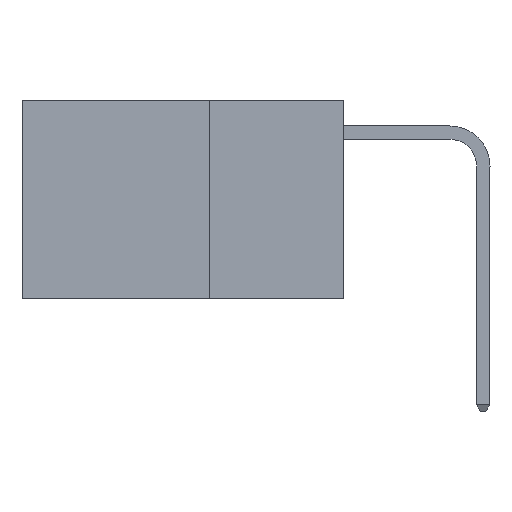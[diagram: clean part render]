
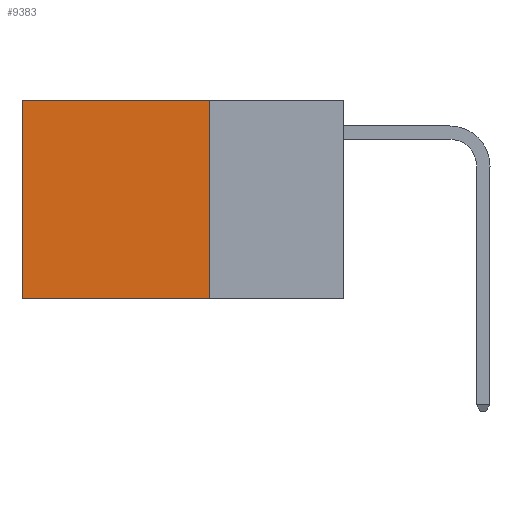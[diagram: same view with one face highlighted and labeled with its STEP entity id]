
A CAD part, left-side view. The second image highlights one B-rep face of the part: STEP entity #9383.
In plain terms, the highlighted planar face has unit normal (-1, 0, 0).
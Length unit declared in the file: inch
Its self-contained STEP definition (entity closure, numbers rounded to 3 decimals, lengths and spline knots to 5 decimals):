
#679 = CARTESIAN_POINT ( 'NONE',  ( 0.2625, 0.25, -0.37 ) ) ;
#1135 = VECTOR ( 'NONE', #7109, 39.37008 ) ;
#1164 = VERTEX_POINT ( 'NONE', #5361 ) ;
#1735 = DIRECTION ( 'NONE',  ( 0., 1., 0. ) ) ;
#1795 = CARTESIAN_POINT ( 'NONE',  ( 0.2625, 0.25, 0. ) ) ;
#3793 = ORIENTED_EDGE ( 'NONE', *, *, #11701, .F. ) ;
#4060 = VECTOR ( 'NONE', #1735, 39.37008 ) ;
#4200 = CARTESIAN_POINT ( 'NONE',  ( 0.2625, 0.25, -0.37 ) ) ;
#4463 = CARTESIAN_POINT ( 'NONE',  ( 0.2625, 0.25, 0. ) ) ;
#4546 = ORIENTED_EDGE ( 'NONE', *, *, #11304, .T. ) ;
#4791 = LINE ( 'NONE', #1795, #4060 ) ;
#5361 = CARTESIAN_POINT ( 'NONE',  ( 0.2625, 0.6, -0.37 ) ) ;
#5553 = CARTESIAN_POINT ( 'NONE',  ( 0.2625, 0.6, 0. ) ) ;
#5702 = FACE_OUTER_BOUND ( 'NONE', #10223, .T. ) ;
#5742 = PLANE ( 'NONE',  #12553 ) ;
#6445 = LINE ( 'NONE', #14404, #10274 ) ;
#7109 = DIRECTION ( 'NONE',  ( 0., 0., -1. ) ) ;
#7186 = CARTESIAN_POINT ( 'NONE',  ( 0.2625, 0.25, 0. ) ) ;
#7611 = VERTEX_POINT ( 'NONE', #5553 ) ;
#7677 = VECTOR ( 'NONE', #11231, 39.37008 ) ;
#7749 = LINE ( 'NONE', #4200, #7677 ) ;
#8507 = DIRECTION ( 'NONE',  ( 1., 0., 0. ) ) ;
#8805 = VERTEX_POINT ( 'NONE', #4463 ) ;
#9212 = EDGE_CURVE ( 'NONE', #9236, #1164, #7749, .T. ) ;
#9236 = VERTEX_POINT ( 'NONE', #679 ) ;
#9383 = ADVANCED_FACE ( 'NONE', ( #5702 ), #5742, .F. ) ;
#9998 = LINE ( 'NONE', #7186, #1135 ) ;
#10223 = EDGE_LOOP ( 'NONE', ( #4546, #12192, #3793, #14560 ) ) ;
#10274 = VECTOR ( 'NONE', #14372, 39.37008 ) ;
#11231 = DIRECTION ( 'NONE',  ( 0., 1., 0. ) ) ;
#11304 = EDGE_CURVE ( 'NONE', #7611, #1164, #6445, .T. ) ;
#11701 = EDGE_CURVE ( 'NONE', #8805, #9236, #9998, .T. ) ;
#12062 = EDGE_CURVE ( 'NONE', #8805, #7611, #4791, .T. ) ;
#12192 = ORIENTED_EDGE ( 'NONE', *, *, #9212, .F. ) ;
#12326 = DIRECTION ( 'NONE',  ( 0., 0., -1. ) ) ;
#12553 = AXIS2_PLACEMENT_3D ( 'NONE', #13065, #8507, #12326 ) ;
#13065 = CARTESIAN_POINT ( 'NONE',  ( 0.2625, 0.25, 0. ) ) ;
#14372 = DIRECTION ( 'NONE',  ( 0., 0., -1. ) ) ;
#14404 = CARTESIAN_POINT ( 'NONE',  ( 0.2625, 0.6, 0. ) ) ;
#14560 = ORIENTED_EDGE ( 'NONE', *, *, #12062, .T. ) ;
